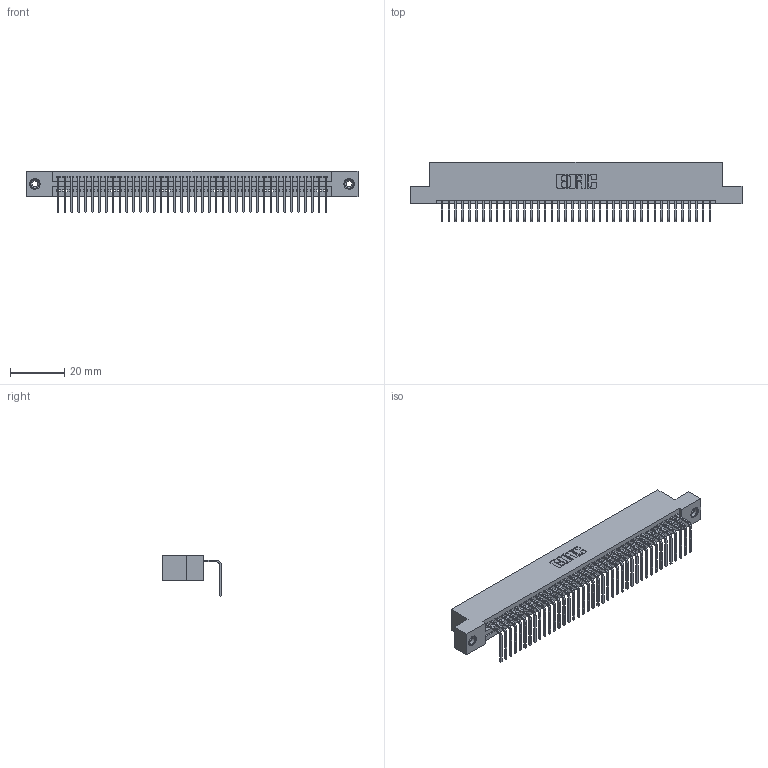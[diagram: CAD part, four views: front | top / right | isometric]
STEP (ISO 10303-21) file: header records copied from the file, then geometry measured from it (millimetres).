
FILE_DESCRIPTION (( 'STEP AP203' ), '1' );
FILE_NAME ('345-040-558-108.STEP', '2019-10-10T16:01:56', ( '' ), ( '' ), 'SwSTEP 2.0', 'SolidWorks 2016', '' );
FILE_SCHEMA (( 'CONFIG_CONTROL_DESIGN' ));
Length unit declared in the file: inch
Products named in the file (4): 345-040-558-108; 345 Part_Flush Mounting Lugs - 0.156 Dia-TI; 345-292-001_558 Tail - 2; 345-250-001_345-250-003-102
Assembly tree (43 placements, depth 2):
  345-040-558-108
    345 Part_Flush Mounting Lugs - 0.156 Dia-TI
    345-292-001_558 Tail - 2  x40
    345-250-001_345-250-003-102  x2
Bounding box: 122.81 x 21.83 x 15.37 mm (x, y, z)
Volume: 11774.9 mm3; surface area: 16422.9 mm2
Topology: 43 solids, 43 shells, 2586 faces, 7757 edges, 5110 vertices
Faces by surface type: plane 1792, cylinder 778, cone 12, torus 4
Entity records: 31644 total; most frequent: CARTESIAN_POINT 5463, ORIENTED_EDGE 5430, DIRECTION 4801, EDGE_CURVE 2715, LINE 2403, VECTOR 2403, VERTEX_POINT 1804, AXIS2_PLACEMENT_3D 1199
